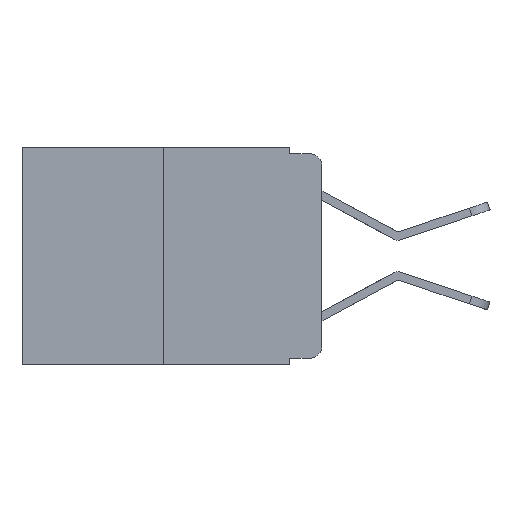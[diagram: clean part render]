
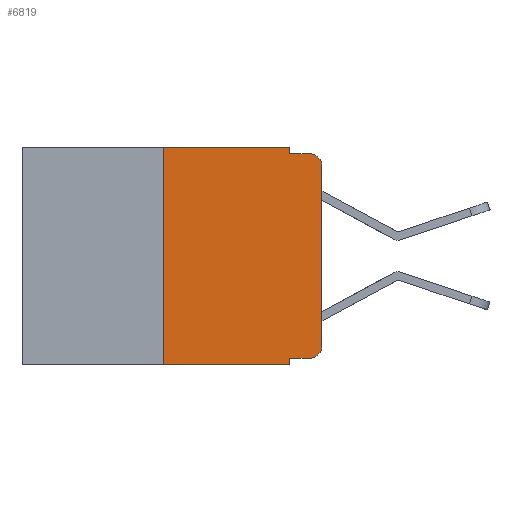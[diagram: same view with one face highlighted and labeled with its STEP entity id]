
A CAD part, left-side view. The second image highlights one B-rep face of the part: STEP entity #6819.
In plain terms, the highlighted planar face has unit normal (-1, 0, 0).
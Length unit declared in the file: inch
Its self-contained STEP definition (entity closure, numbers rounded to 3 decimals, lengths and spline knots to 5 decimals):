
#455 = VECTOR ( 'NONE', #8519, 39.37008 ) ;
#526 = EDGE_CURVE ( 'NONE', #13435, #12807, #10547, .T. ) ;
#800 = PLANE ( 'NONE',  #12356 ) ;
#1550 = DIRECTION ( 'NONE',  ( 0., -1., 0. ) ) ;
#2182 = CARTESIAN_POINT ( 'NONE',  ( 0., 0.02, -0.03 ) ) ;
#2464 = EDGE_CURVE ( 'NONE', #6225, #12374, #14127, .T. ) ;
#2592 = DIRECTION ( 'NONE',  ( 0., -1., 0. ) ) ;
#2675 = CARTESIAN_POINT ( 'NONE',  ( 0., 0.051, -0.343 ) ) ;
#2930 = CARTESIAN_POINT ( 'NONE',  ( 0., 0.051, -0.333 ) ) ;
#2996 = ORIENTED_EDGE ( 'NONE', *, *, #11110, .F. ) ;
#3191 = CARTESIAN_POINT ( 'NONE',  ( 0., 0.051, 0. ) ) ;
#3207 = CARTESIAN_POINT ( 'NONE',  ( 0., 0.25, 0. ) ) ;
#3240 = CARTESIAN_POINT ( 'NONE',  ( 0., 0.051, -0.01 ) ) ;
#3414 = DIRECTION ( 'NONE',  ( 0., 0., 1. ) ) ;
#3734 = CARTESIAN_POINT ( 'NONE',  ( 0., 0.25, -0.343 ) ) ;
#3773 = AXIS2_PLACEMENT_3D ( 'NONE', #4115, #5314, #15808 ) ;
#3910 = LINE ( 'NONE', #3191, #455 ) ;
#4028 = VERTEX_POINT ( 'NONE', #6049 ) ;
#4044 = ORIENTED_EDGE ( 'NONE', *, *, #13044, .T. ) ;
#4115 = CARTESIAN_POINT ( 'NONE',  ( 0., 0.02, -0.313 ) ) ;
#4218 = FACE_OUTER_BOUND ( 'NONE', #10461, .T. ) ;
#4282 = LINE ( 'NONE', #13840, #6334 ) ;
#4321 = CARTESIAN_POINT ( 'NONE',  ( 0., 0.051, 0. ) ) ;
#4503 = LINE ( 'NONE', #3240, #15728 ) ;
#4699 = DIRECTION ( 'NONE',  ( 0., 0., 1. ) ) ;
#4706 = EDGE_CURVE ( 'NONE', #6498, #13435, #7542, .T. ) ;
#4918 = CARTESIAN_POINT ( 'NONE',  ( 0., 0.02, -0.01 ) ) ;
#4964 = EDGE_CURVE ( 'NONE', #10017, #13247, #7330, .T. ) ;
#5117 = VERTEX_POINT ( 'NONE', #2675 ) ;
#5146 = LINE ( 'NONE', #4321, #16364 ) ;
#5305 = LINE ( 'NONE', #8196, #7129 ) ;
#5314 = DIRECTION ( 'NONE',  ( -1., 0., 0. ) ) ;
#5359 = CARTESIAN_POINT ( 'NONE',  ( 0., 0.02, -0.333 ) ) ;
#5376 = ORIENTED_EDGE ( 'NONE', *, *, #11443, .F. ) ;
#6049 = CARTESIAN_POINT ( 'NONE',  ( 0., 0.051, -0.01 ) ) ;
#6065 = CARTESIAN_POINT ( 'NONE',  ( 0., 0., -0.03 ) ) ;
#6091 = DIRECTION ( 'NONE',  ( -1., 0., 0. ) ) ;
#6225 = VERTEX_POINT ( 'NONE', #6065 ) ;
#6334 = VECTOR ( 'NONE', #3414, 39.37008 ) ;
#6498 = VERTEX_POINT ( 'NONE', #15190 ) ;
#6819 = ADVANCED_FACE ( 'NONE', ( #4218 ), #800, .F. ) ;
#7129 = VECTOR ( 'NONE', #1550, 39.37008 ) ;
#7278 = ORIENTED_EDGE ( 'NONE', *, *, #2464, .T. ) ;
#7330 = LINE ( 'NONE', #3207, #12215 ) ;
#7542 = LINE ( 'NONE', #2930, #15309 ) ;
#8196 = CARTESIAN_POINT ( 'NONE',  ( 0., 0.473, 0. ) ) ;
#8519 = DIRECTION ( 'NONE',  ( 0., 0., -1. ) ) ;
#8903 = DIRECTION ( 'NONE',  ( 1., 0., 0. ) ) ;
#9058 = CARTESIAN_POINT ( 'NONE',  ( 0., 0.473, -0.343 ) ) ;
#9210 = ORIENTED_EDGE ( 'NONE', *, *, #13628, .F. ) ;
#9713 = ORIENTED_EDGE ( 'NONE', *, *, #10453, .F. ) ;
#10017 = VERTEX_POINT ( 'NONE', #3734 ) ;
#10229 = ORIENTED_EDGE ( 'NONE', *, *, #526, .T. ) ;
#10453 = EDGE_CURVE ( 'NONE', #14198, #4028, #3910, .T. ) ;
#10461 = EDGE_LOOP ( 'NONE', ( #14597, #7278, #2996, #9713, #5376, #16747, #4044, #9210, #12863, #10229 ) ) ;
#10470 = LINE ( 'NONE', #9058, #15965 ) ;
#10534 = CARTESIAN_POINT ( 'NONE',  ( 0., 0.051, 0. ) ) ;
#10547 = CIRCLE ( 'NONE', #3773, 0.02 ) ;
#10666 = DIRECTION ( 'NONE',  ( 0., 0., -1. ) ) ;
#10881 = CARTESIAN_POINT ( 'NONE',  ( 0., 0., -0.313 ) ) ;
#11061 = EDGE_CURVE ( 'NONE', #12807, #6225, #4282, .T. ) ;
#11108 = DIRECTION ( 'NONE',  ( 0., -1., 0. ) ) ;
#11110 = EDGE_CURVE ( 'NONE', #4028, #12374, #4503, .T. ) ;
#11443 = EDGE_CURVE ( 'NONE', #13247, #14198, #5305, .T. ) ;
#11523 = CARTESIAN_POINT ( 'NONE',  ( 0., 0.25, 0. ) ) ;
#12159 = DIRECTION ( 'NONE',  ( 0., -1., 0. ) ) ;
#12215 = VECTOR ( 'NONE', #4699, 39.37008 ) ;
#12350 = DIRECTION ( 'NONE',  ( 0., 0., -1. ) ) ;
#12356 = AXIS2_PLACEMENT_3D ( 'NONE', #12526, #8903, #12350 ) ;
#12374 = VERTEX_POINT ( 'NONE', #4918 ) ;
#12526 = CARTESIAN_POINT ( 'NONE',  ( 0., 0.473, 0. ) ) ;
#12807 = VERTEX_POINT ( 'NONE', #10881 ) ;
#12863 = ORIENTED_EDGE ( 'NONE', *, *, #4706, .T. ) ;
#13044 = EDGE_CURVE ( 'NONE', #10017, #5117, #10470, .T. ) ;
#13247 = VERTEX_POINT ( 'NONE', #11523 ) ;
#13435 = VERTEX_POINT ( 'NONE', #5359 ) ;
#13628 = EDGE_CURVE ( 'NONE', #6498, #5117, #5146, .T. ) ;
#13728 = AXIS2_PLACEMENT_3D ( 'NONE', #2182, #6091, #16621 ) ;
#13840 = CARTESIAN_POINT ( 'NONE',  ( 0., 0., 0. ) ) ;
#14127 = CIRCLE ( 'NONE', #13728, 0.02 ) ;
#14198 = VERTEX_POINT ( 'NONE', #10534 ) ;
#14597 = ORIENTED_EDGE ( 'NONE', *, *, #11061, .T. ) ;
#15190 = CARTESIAN_POINT ( 'NONE',  ( 0., 0.051, -0.333 ) ) ;
#15309 = VECTOR ( 'NONE', #12159, 39.37008 ) ;
#15728 = VECTOR ( 'NONE', #11108, 39.37008 ) ;
#15808 = DIRECTION ( 'NONE',  ( 0., 0., -1. ) ) ;
#15965 = VECTOR ( 'NONE', #2592, 39.37008 ) ;
#16364 = VECTOR ( 'NONE', #10666, 39.37008 ) ;
#16621 = DIRECTION ( 'NONE',  ( 0., 0., -1. ) ) ;
#16747 = ORIENTED_EDGE ( 'NONE', *, *, #4964, .F. ) ;
